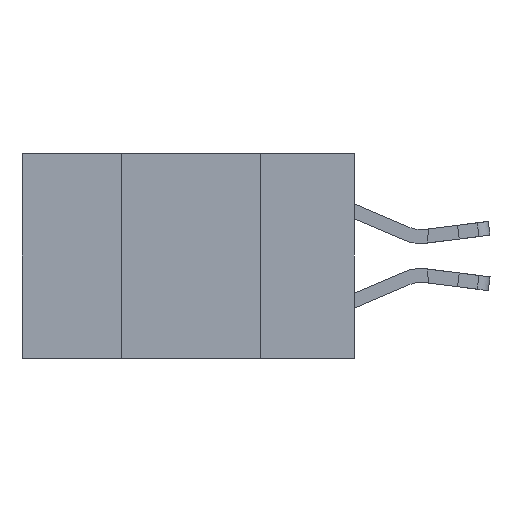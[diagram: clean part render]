
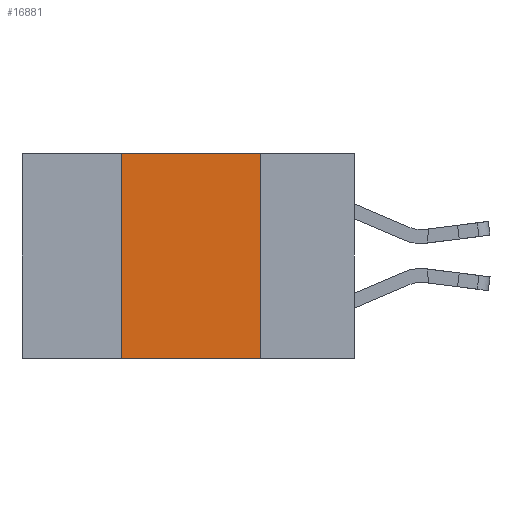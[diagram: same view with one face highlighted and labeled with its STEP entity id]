
A CAD part, left-side view. The second image highlights one B-rep face of the part: STEP entity #16881.
In plain terms, the highlighted planar face has unit normal (-1, 0, 0).
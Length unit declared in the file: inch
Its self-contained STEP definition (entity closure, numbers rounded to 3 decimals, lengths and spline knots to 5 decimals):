
#631 = PLANE ( 'NONE',  #15555 ) ;
#2051 = LINE ( 'NONE', #4842, #19609 ) ;
#2374 = DIRECTION ( 'NONE',  ( 0., 0., -1. ) ) ;
#2803 = CARTESIAN_POINT ( 'NONE',  ( 0., 0.17, -0.37 ) ) ;
#3205 = EDGE_CURVE ( 'NONE', #21095, #10980, #10906, .T. ) ;
#3713 = DIRECTION ( 'NONE',  ( 0., 0., 1. ) ) ;
#4842 = CARTESIAN_POINT ( 'NONE',  ( 0., 0.6, -0.37 ) ) ;
#4951 = CARTESIAN_POINT ( 'NONE',  ( 0., 0.17, 0. ) ) ;
#5778 = CARTESIAN_POINT ( 'NONE',  ( 0., 0.6, 0. ) ) ;
#6230 = VERTEX_POINT ( 'NONE', #4951 ) ;
#6600 = ORIENTED_EDGE ( 'NONE', *, *, #19134, .F. ) ;
#7545 = VECTOR ( 'NONE', #13693, 39.37008 ) ;
#8309 = ORIENTED_EDGE ( 'NONE', *, *, #14683, .F. ) ;
#8906 = ORIENTED_EDGE ( 'NONE', *, *, #19270, .T. ) ;
#9036 = CARTESIAN_POINT ( 'NONE',  ( 0., 0.42, -0.37 ) ) ;
#9336 = CARTESIAN_POINT ( 'NONE',  ( 0., 0.42, 0. ) ) ;
#10225 = VERTEX_POINT ( 'NONE', #14225 ) ;
#10906 = LINE ( 'NONE', #15676, #11451 ) ;
#10980 = VERTEX_POINT ( 'NONE', #9336 ) ;
#11451 = VECTOR ( 'NONE', #3713, 39.37008 ) ;
#11990 = CARTESIAN_POINT ( 'NONE',  ( 0., 0.6, 0. ) ) ;
#12658 = DIRECTION ( 'NONE',  ( 1., 0., 0. ) ) ;
#13693 = DIRECTION ( 'NONE',  ( 0., -1., 0. ) ) ;
#14225 = CARTESIAN_POINT ( 'NONE',  ( 0., 0.17, -0.37 ) ) ;
#14683 = EDGE_CURVE ( 'NONE', #10980, #6230, #16573, .T. ) ;
#14798 = DIRECTION ( 'NONE',  ( 0., 0., -1. ) ) ;
#15555 = AXIS2_PLACEMENT_3D ( 'NONE', #5778, #12658, #2374 ) ;
#15676 = CARTESIAN_POINT ( 'NONE',  ( 0., 0.42, -0.37 ) ) ;
#16573 = LINE ( 'NONE', #11990, #7545 ) ;
#16881 = ADVANCED_FACE ( 'NONE', ( #16977 ), #631, .F. ) ;
#16977 = FACE_OUTER_BOUND ( 'NONE', #21048, .T. ) ;
#17802 = VECTOR ( 'NONE', #14798, 39.37008 ) ;
#18307 = LINE ( 'NONE', #2803, #17802 ) ;
#18424 = DIRECTION ( 'NONE',  ( 0., -1., 0. ) ) ;
#19134 = EDGE_CURVE ( 'NONE', #6230, #10225, #18307, .T. ) ;
#19270 = EDGE_CURVE ( 'NONE', #21095, #10225, #2051, .T. ) ;
#19609 = VECTOR ( 'NONE', #18424, 39.37008 ) ;
#21048 = EDGE_LOOP ( 'NONE', ( #6600, #8309, #21649, #8906 ) ) ;
#21095 = VERTEX_POINT ( 'NONE', #9036 ) ;
#21649 = ORIENTED_EDGE ( 'NONE', *, *, #3205, .F. ) ;
